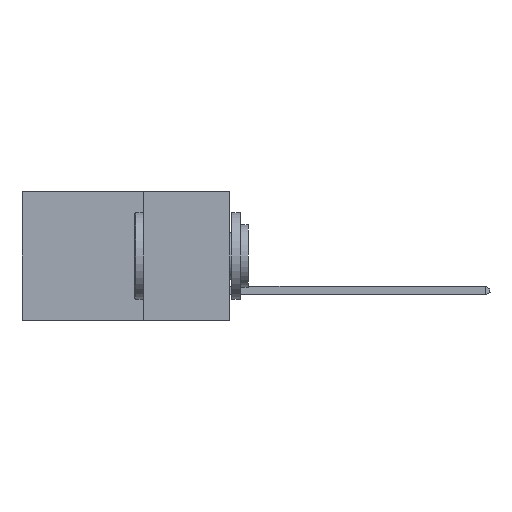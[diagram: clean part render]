
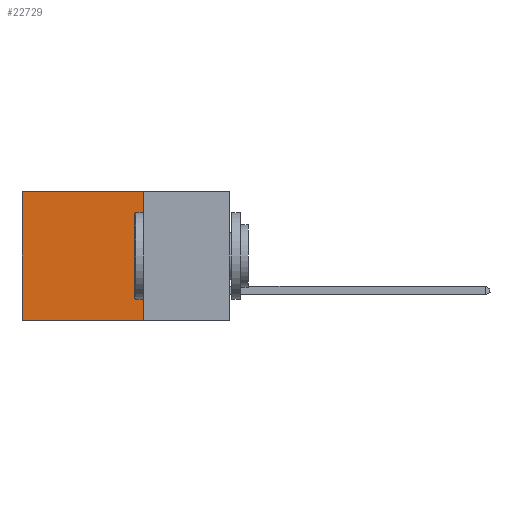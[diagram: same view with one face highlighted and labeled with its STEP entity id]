
A CAD part, left-side view. The second image highlights one B-rep face of the part: STEP entity #22729.
In plain terms, the highlighted planar face has unit normal (-1, 0, 0).
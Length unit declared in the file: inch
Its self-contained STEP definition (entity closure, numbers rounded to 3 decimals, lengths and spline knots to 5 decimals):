
#44 = DIRECTION ( 'NONE',  ( 0., 0., -1. ) ) ;
#937 = ORIENTED_EDGE ( 'NONE', *, *, #4500, .F. ) ;
#2351 = LINE ( 'NONE', #27073, #19645 ) ;
#2979 = CARTESIAN_POINT ( 'NONE',  ( 0.298, 0.25, -0.37 ) ) ;
#3096 = CARTESIAN_POINT ( 'NONE',  ( 0.298, 0.6, -0.37 ) ) ;
#3171 = FACE_OUTER_BOUND ( 'NONE', #11839, .T. ) ;
#3298 = VECTOR ( 'NONE', #3792, 39.37008 ) ;
#3499 = CARTESIAN_POINT ( 'NONE',  ( 0.298, 0.25, 0. ) ) ;
#3792 = DIRECTION ( 'NONE',  ( 0., 0., -1. ) ) ;
#3899 = PLANE ( 'NONE',  #28711 ) ;
#4500 = EDGE_CURVE ( 'NONE', #26461, #8928, #16021, .T. ) ;
#4987 = CARTESIAN_POINT ( 'NONE',  ( 0.298, 0.25, 0. ) ) ;
#4993 = CARTESIAN_POINT ( 'NONE',  ( 0.298, 0.25, -0.37 ) ) ;
#6727 = ORIENTED_EDGE ( 'NONE', *, *, #7418, .F. ) ;
#7418 = EDGE_CURVE ( 'NONE', #8928, #14548, #23698, .T. ) ;
#8422 = DIRECTION ( 'NONE',  ( 0., 0., -1. ) ) ;
#8928 = VERTEX_POINT ( 'NONE', #2979 ) ;
#10404 = VERTEX_POINT ( 'NONE', #12853 ) ;
#11839 = EDGE_LOOP ( 'NONE', ( #23978, #6727, #937, #27937 ) ) ;
#12127 = DIRECTION ( 'NONE',  ( 0., 1., 0. ) ) ;
#12853 = CARTESIAN_POINT ( 'NONE',  ( 0.298, 0.6, 0. ) ) ;
#14548 = VERTEX_POINT ( 'NONE', #3096 ) ;
#16021 = LINE ( 'NONE', #3499, #3298 ) ;
#17107 = EDGE_CURVE ( 'NONE', #10404, #14548, #2351, .T. ) ;
#17752 = VECTOR ( 'NONE', #27559, 39.37008 ) ;
#19645 = VECTOR ( 'NONE', #44, 39.37008 ) ;
#19721 = CARTESIAN_POINT ( 'NONE',  ( 0.298, 0.25, 0. ) ) ;
#20479 = EDGE_CURVE ( 'NONE', #26461, #10404, #28361, .T. ) ;
#21968 = DIRECTION ( 'NONE',  ( 1., 0., 0. ) ) ;
#22382 = VECTOR ( 'NONE', #12127, 39.37008 ) ;
#22729 = ADVANCED_FACE ( 'NONE', ( #3171 ), #3899, .F. ) ;
#23698 = LINE ( 'NONE', #4993, #17752 ) ;
#23978 = ORIENTED_EDGE ( 'NONE', *, *, #17107, .T. ) ;
#26461 = VERTEX_POINT ( 'NONE', #4987 ) ;
#27073 = CARTESIAN_POINT ( 'NONE',  ( 0.298, 0.6, 0. ) ) ;
#27559 = DIRECTION ( 'NONE',  ( 0., 1., 0. ) ) ;
#27621 = CARTESIAN_POINT ( 'NONE',  ( 0.298, 0.25, 0. ) ) ;
#27937 = ORIENTED_EDGE ( 'NONE', *, *, #20479, .T. ) ;
#28361 = LINE ( 'NONE', #27621, #22382 ) ;
#28711 = AXIS2_PLACEMENT_3D ( 'NONE', #19721, #21968, #8422 ) ;
